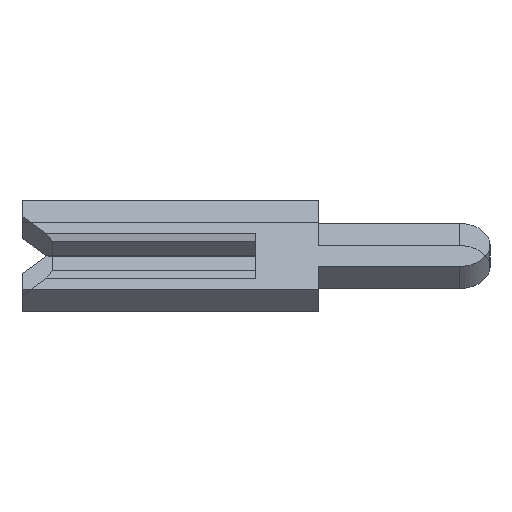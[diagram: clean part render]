
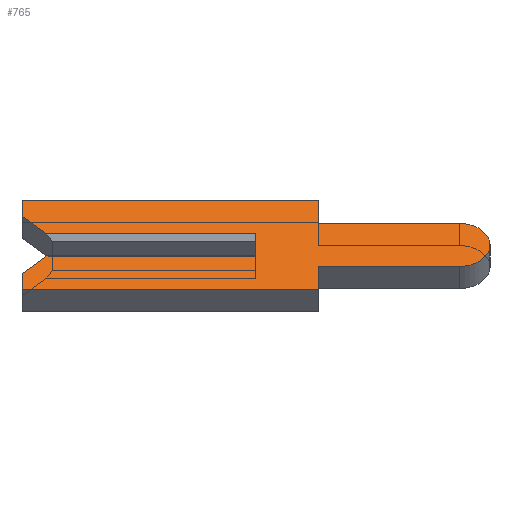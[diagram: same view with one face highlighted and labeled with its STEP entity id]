
A CAD part, left-side view. The second image highlights one B-rep face of the part: STEP entity #765.
In plain terms, the highlighted face is planar.
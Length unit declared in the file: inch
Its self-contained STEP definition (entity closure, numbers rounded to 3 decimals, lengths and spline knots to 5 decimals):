
#9 = CARTESIAN_POINT ( 'NONE',  ( -0.01, -0.04, -0.0195 ) ) ;
#34 = VECTOR ( 'NONE', #701, 39.37008 ) ;
#65 = EDGE_CURVE ( 'NONE', #1578, #919, #1064, .T. ) ;
#84 = LINE ( 'NONE', #9, #372 ) ;
#108 = VECTOR ( 'NONE', #2385, 39.37008 ) ;
#193 = LINE ( 'NONE', #369, #1686 ) ;
#233 = ORIENTED_EDGE ( 'NONE', *, *, #412, .F. ) ;
#241 = CARTESIAN_POINT ( 'NONE',  ( -0.01, 0.15, -0.026 ) ) ;
#247 = DIRECTION ( 'NONE',  ( 0., 0., -1. ) ) ;
#263 = PLANE ( 'NONE',  #570 ) ;
#275 = LINE ( 'NONE', #2129, #108 ) ;
#276 = DIRECTION ( 'NONE',  ( 0., 1., 0. ) ) ;
#287 = EDGE_CURVE ( 'NONE', #514, #2833, #684, .T. ) ;
#292 = VERTEX_POINT ( 'NONE', #1741 ) ;
#332 = CARTESIAN_POINT ( 'NONE',  ( -0.01, 0., 0.01 ) ) ;
#369 = CARTESIAN_POINT ( 'NONE',  ( -0.01, -0.1305, -0.01 ) ) ;
#372 = VECTOR ( 'NONE', #276, 39.37008 ) ;
#399 = DIRECTION ( 'NONE',  ( 0., 0., -1. ) ) ;
#407 = LINE ( 'NONE', #813, #3186 ) ;
#412 = EDGE_CURVE ( 'NONE', #1909, #1842, #84, .T. ) ;
#492 = VECTOR ( 'NONE', #838, 39.37008 ) ;
#514 = VERTEX_POINT ( 'NONE', #528 ) ;
#526 = EDGE_CURVE ( 'NONE', #2833, #1413, #2639, .T. ) ;
#528 = CARTESIAN_POINT ( 'NONE',  ( -0.01, 0.15, 0.026 ) ) ;
#570 = AXIS2_PLACEMENT_3D ( 'NONE', #1559, #2781, #247 ) ;
#596 = CARTESIAN_POINT ( 'NONE',  ( -0.01, -0.1305, -0.0195 ) ) ;
#606 = LINE ( 'NONE', #2258, #643 ) ;
#630 = EDGE_CURVE ( 'NONE', #1680, #514, #1493, .T. ) ;
#643 = VECTOR ( 'NONE', #997, 39.37008 ) ;
#684 = LINE ( 'NONE', #730, #2229 ) ;
#701 = DIRECTION ( 'NONE',  ( 0., -1., 0. ) ) ;
#730 = CARTESIAN_POINT ( 'NONE',  ( -0.01, 0.15, 0.026 ) ) ;
#739 = CARTESIAN_POINT ( 'NONE',  ( -0.01, 0., -0.01 ) ) ;
#745 = DIRECTION ( 'NONE',  ( 1., 0., 0. ) ) ;
#765 = ADVANCED_FACE ( 'NONE', ( #1772 ), #263, .F. ) ;
#802 = EDGE_CURVE ( 'NONE', #1190, #1909, #1689, .T. ) ;
#813 = CARTESIAN_POINT ( 'NONE',  ( -0.01, -0.04, 0.04 ) ) ;
#838 = DIRECTION ( 'NONE',  ( 0., 0., 1. ) ) ;
#839 = ORIENTED_EDGE ( 'NONE', *, *, #1276, .T. ) ;
#919 = VERTEX_POINT ( 'NONE', #241 ) ;
#969 = ORIENTED_EDGE ( 'NONE', *, *, #2984, .F. ) ;
#997 = DIRECTION ( 'NONE',  ( 0., -0.707, 0.707 ) ) ;
#1016 = DIRECTION ( 'NONE',  ( 0., 0., -1. ) ) ;
#1039 = CARTESIAN_POINT ( 'NONE',  ( -0.01, -0.1305, 0. ) ) ;
#1064 = LINE ( 'NONE', #2249, #3229 ) ;
#1094 = CARTESIAN_POINT ( 'NONE',  ( -0.01, 0.15, 0.01 ) ) ;
#1110 = CARTESIAN_POINT ( 'NONE',  ( -0.01, 0.15, -0.04 ) ) ;
#1151 = CARTESIAN_POINT ( 'NONE',  ( -0.01, 0.134, -0.01 ) ) ;
#1167 = VECTOR ( 'NONE', #2356, 39.37008 ) ;
#1190 = VERTEX_POINT ( 'NONE', #1290 ) ;
#1251 = LINE ( 'NONE', #1837, #492 ) ;
#1276 = EDGE_CURVE ( 'NONE', #1680, #1283, #1992, .T. ) ;
#1283 = VERTEX_POINT ( 'NONE', #332 ) ;
#1290 = CARTESIAN_POINT ( 'NONE',  ( -0.01, -0.1305, 0.0195 ) ) ;
#1312 = DIRECTION ( 'NONE',  ( 0., 0.707, 0.707 ) ) ;
#1368 = LINE ( 'NONE', #2790, #34 ) ;
#1385 = CARTESIAN_POINT ( 'NONE',  ( -0.01, -0.04, -0.0195 ) ) ;
#1413 = VERTEX_POINT ( 'NONE', #2600 ) ;
#1436 = ORIENTED_EDGE ( 'NONE', *, *, #2453, .F. ) ;
#1442 = CARTESIAN_POINT ( 'NONE',  ( -0.01, 0.15, 0.04 ) ) ;
#1447 = EDGE_CURVE ( 'NONE', #3138, #1283, #1251, .T. ) ;
#1469 = AXIS2_PLACEMENT_3D ( 'NONE', #1039, #745, #1016 ) ;
#1493 = LINE ( 'NONE', #2017, #1890 ) ;
#1511 = EDGE_CURVE ( 'NONE', #1413, #292, #407, .T. ) ;
#1526 = EDGE_LOOP ( 'NONE', ( #839, #1755, #2945, #969, #2586, #1436, #2064, #233, #2211, #1805, #2457, #3107, #2295, #3034 ) ) ;
#1559 = CARTESIAN_POINT ( 'NONE',  ( -0.01, -0.1305, 0. ) ) ;
#1578 = VERTEX_POINT ( 'NONE', #1110 ) ;
#1606 = DIRECTION ( 'NONE',  ( 0., 0., -1. ) ) ;
#1680 = VERTEX_POINT ( 'NONE', #2100 ) ;
#1686 = VECTOR ( 'NONE', #2376, 39.37008 ) ;
#1689 = CIRCLE ( 'NONE', #1469, 0.0195 ) ;
#1741 = CARTESIAN_POINT ( 'NONE',  ( -0.01, -0.04, 0.0195 ) ) ;
#1755 = ORIENTED_EDGE ( 'NONE', *, *, #1447, .F. ) ;
#1772 = FACE_OUTER_BOUND ( 'NONE', #1526, .T. ) ;
#1805 = ORIENTED_EDGE ( 'NONE', *, *, #3221, .F. ) ;
#1837 = CARTESIAN_POINT ( 'NONE',  ( -0.01, 0., 0.0065 ) ) ;
#1842 = VERTEX_POINT ( 'NONE', #1385 ) ;
#1890 = VECTOR ( 'NONE', #1312, 39.37008 ) ;
#1909 = VERTEX_POINT ( 'NONE', #596 ) ;
#1953 = VECTOR ( 'NONE', #2310, 39.37008 ) ;
#1986 = DIRECTION ( 'NONE',  ( 0., 0., 1. ) ) ;
#1992 = LINE ( 'NONE', #1094, #1167 ) ;
#2017 = CARTESIAN_POINT ( 'NONE',  ( -0.01, 0.1305, 0.0065 ) ) ;
#2064 = ORIENTED_EDGE ( 'NONE', *, *, #2561, .F. ) ;
#2100 = CARTESIAN_POINT ( 'NONE',  ( -0.01, 0.134, 0.01 ) ) ;
#2129 = CARTESIAN_POINT ( 'NONE',  ( -0.01, 0.15, -0.04 ) ) ;
#2211 = ORIENTED_EDGE ( 'NONE', *, *, #802, .F. ) ;
#2213 = EDGE_CURVE ( 'NONE', #2259, #3138, #193, .T. ) ;
#2229 = VECTOR ( 'NONE', #3022, 39.37008 ) ;
#2249 = CARTESIAN_POINT ( 'NONE',  ( -0.01, 0.15, -0.026 ) ) ;
#2258 = CARTESIAN_POINT ( 'NONE',  ( -0.01, 0.1305, -0.0065 ) ) ;
#2259 = VERTEX_POINT ( 'NONE', #1151 ) ;
#2282 = CARTESIAN_POINT ( 'NONE',  ( -0.01, 0.15, 0.04 ) ) ;
#2295 = ORIENTED_EDGE ( 'NONE', *, *, #287, .F. ) ;
#2310 = DIRECTION ( 'NONE',  ( 0., -1., 0. ) ) ;
#2356 = DIRECTION ( 'NONE',  ( 0., -1., 0. ) ) ;
#2376 = DIRECTION ( 'NONE',  ( 0., -1., 0. ) ) ;
#2385 = DIRECTION ( 'NONE',  ( 0., 1., 0. ) ) ;
#2453 = EDGE_CURVE ( 'NONE', #3175, #1578, #275, .T. ) ;
#2457 = ORIENTED_EDGE ( 'NONE', *, *, #1511, .F. ) ;
#2478 = CARTESIAN_POINT ( 'NONE',  ( -0.01, -0.04, -0.04 ) ) ;
#2561 = EDGE_CURVE ( 'NONE', #1842, #3175, #2911, .T. ) ;
#2586 = ORIENTED_EDGE ( 'NONE', *, *, #65, .F. ) ;
#2600 = CARTESIAN_POINT ( 'NONE',  ( -0.01, -0.04, 0.04 ) ) ;
#2639 = LINE ( 'NONE', #2282, #1953 ) ;
#2781 = DIRECTION ( 'NONE',  ( 1., 0., 0. ) ) ;
#2790 = CARTESIAN_POINT ( 'NONE',  ( -0.01, -0.04, 0.0195 ) ) ;
#2833 = VERTEX_POINT ( 'NONE', #1442 ) ;
#2911 = LINE ( 'NONE', #3190, #3222 ) ;
#2945 = ORIENTED_EDGE ( 'NONE', *, *, #2213, .F. ) ;
#2984 = EDGE_CURVE ( 'NONE', #919, #2259, #606, .T. ) ;
#3022 = DIRECTION ( 'NONE',  ( 0., 0., 1. ) ) ;
#3034 = ORIENTED_EDGE ( 'NONE', *, *, #630, .F. ) ;
#3107 = ORIENTED_EDGE ( 'NONE', *, *, #526, .F. ) ;
#3138 = VERTEX_POINT ( 'NONE', #739 ) ;
#3175 = VERTEX_POINT ( 'NONE', #2478 ) ;
#3186 = VECTOR ( 'NONE', #1606, 39.37008 ) ;
#3190 = CARTESIAN_POINT ( 'NONE',  ( -0.01, -0.04, -0.04 ) ) ;
#3221 = EDGE_CURVE ( 'NONE', #292, #1190, #1368, .T. ) ;
#3222 = VECTOR ( 'NONE', #399, 39.37008 ) ;
#3229 = VECTOR ( 'NONE', #1986, 39.37008 ) ;
